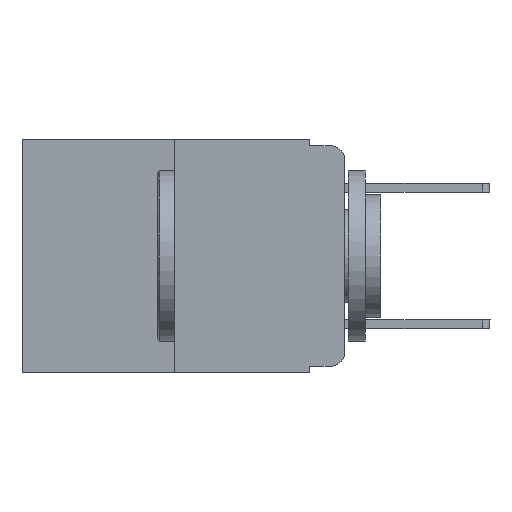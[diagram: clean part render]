
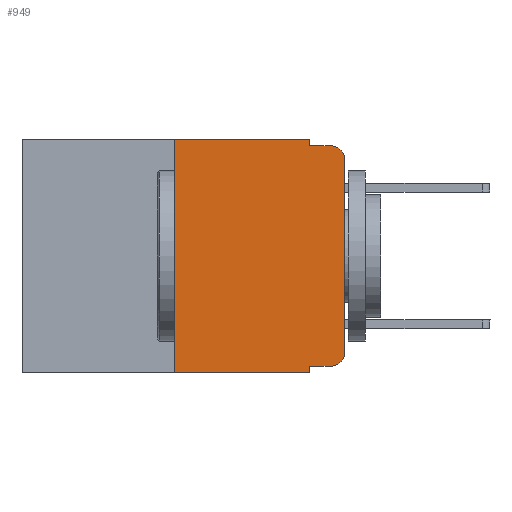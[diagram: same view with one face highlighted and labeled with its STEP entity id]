
A CAD part, left-side view. The second image highlights one B-rep face of the part: STEP entity #949.
In plain terms, the highlighted planar face has unit normal (-1, 0, 0).
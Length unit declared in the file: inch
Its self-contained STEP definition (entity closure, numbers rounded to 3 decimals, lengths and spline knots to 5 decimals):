
#82 = PLANE ( 'NONE',  #6719 ) ;
#690 = CARTESIAN_POINT ( 'NONE',  ( 0., 0.25, 0. ) ) ;
#942 = EDGE_CURVE ( 'NONE', #7728, #4153, #3544, .T. ) ;
#946 = VECTOR ( 'NONE', #10002, 39.37008 ) ;
#949 = ADVANCED_FACE ( 'NONE', ( #10896 ), #82, .F. ) ;
#1170 = VERTEX_POINT ( 'NONE', #7969 ) ;
#1333 = CARTESIAN_POINT ( 'NONE',  ( 0., 0.473, 0. ) ) ;
#1554 = ORIENTED_EDGE ( 'NONE', *, *, #13629, .T. ) ;
#1959 = EDGE_CURVE ( 'NONE', #1170, #15114, #11874, .T. ) ;
#1982 = CARTESIAN_POINT ( 'NONE',  ( 0., 0.02, -0.333 ) ) ;
#2092 = EDGE_CURVE ( 'NONE', #14401, #10902, #7613, .T. ) ;
#2236 = CARTESIAN_POINT ( 'NONE',  ( 0., 0.473, -0.343 ) ) ;
#2256 = ORIENTED_EDGE ( 'NONE', *, *, #4813, .F. ) ;
#2295 = VERTEX_POINT ( 'NONE', #6242 ) ;
#2588 = DIRECTION ( 'NONE',  ( 0., 0., -1. ) ) ;
#2634 = CARTESIAN_POINT ( 'NONE',  ( 0., 0.473, 0. ) ) ;
#2963 = LINE ( 'NONE', #7412, #11364 ) ;
#3075 = VECTOR ( 'NONE', #16510, 39.37008 ) ;
#3254 = CARTESIAN_POINT ( 'NONE',  ( 0., 0.051, -0.01 ) ) ;
#3415 = EDGE_CURVE ( 'NONE', #4444, #14196, #16732, .T. ) ;
#3544 = LINE ( 'NONE', #13118, #12304 ) ;
#3680 = ORIENTED_EDGE ( 'NONE', *, *, #2092, .F. ) ;
#3796 = AXIS2_PLACEMENT_3D ( 'NONE', #14448, #11604, #2588 ) ;
#3921 = EDGE_LOOP ( 'NONE', ( #6752, #1554, #2256, #13914, #3680, #6070, #8173, #13683, #13989, #15368 ) ) ;
#4153 = VERTEX_POINT ( 'NONE', #6490 ) ;
#4444 = VERTEX_POINT ( 'NONE', #15946 ) ;
#4813 = EDGE_CURVE ( 'NONE', #6234, #2295, #2963, .T. ) ;
#5033 = CARTESIAN_POINT ( 'NONE',  ( 0., 0.051, -0.343 ) ) ;
#5127 = CIRCLE ( 'NONE', #14091, 0.02 ) ;
#5692 = VECTOR ( 'NONE', #6187, 39.37008 ) ;
#6070 = ORIENTED_EDGE ( 'NONE', *, *, #13363, .F. ) ;
#6122 = DIRECTION ( 'NONE',  ( -1., 0., 0. ) ) ;
#6187 = DIRECTION ( 'NONE',  ( 0., -1., 0. ) ) ;
#6234 = VERTEX_POINT ( 'NONE', #3254 ) ;
#6242 = CARTESIAN_POINT ( 'NONE',  ( 0., 0.02, -0.01 ) ) ;
#6354 = DIRECTION ( 'NONE',  ( 0., 0., -1. ) ) ;
#6490 = CARTESIAN_POINT ( 'NONE',  ( 0., 0., -0.03 ) ) ;
#6719 = AXIS2_PLACEMENT_3D ( 'NONE', #1333, #11689, #10480 ) ;
#6752 = ORIENTED_EDGE ( 'NONE', *, *, #942, .T. ) ;
#6802 = LINE ( 'NONE', #9765, #16832 ) ;
#7412 = CARTESIAN_POINT ( 'NONE',  ( 0., 0.051, -0.01 ) ) ;
#7445 = CARTESIAN_POINT ( 'NONE',  ( 0., 0.02, -0.313 ) ) ;
#7564 = CARTESIAN_POINT ( 'NONE',  ( 0., 0.051, 0. ) ) ;
#7613 = LINE ( 'NONE', #2634, #3075 ) ;
#7728 = VERTEX_POINT ( 'NONE', #14671 ) ;
#7969 = CARTESIAN_POINT ( 'NONE',  ( 0., 0.051, -0.333 ) ) ;
#8173 = ORIENTED_EDGE ( 'NONE', *, *, #3415, .T. ) ;
#8855 = DIRECTION ( 'NONE',  ( 0., -1., 0. ) ) ;
#9109 = LINE ( 'NONE', #690, #946 ) ;
#9646 = EDGE_CURVE ( 'NONE', #1170, #14196, #6802, .T. ) ;
#9765 = CARTESIAN_POINT ( 'NONE',  ( 0., 0.051, 0. ) ) ;
#10002 = DIRECTION ( 'NONE',  ( 0., 0., 1. ) ) ;
#10020 = CARTESIAN_POINT ( 'NONE',  ( 0., 0.051, 0. ) ) ;
#10300 = EDGE_CURVE ( 'NONE', #10902, #6234, #16820, .T. ) ;
#10480 = DIRECTION ( 'NONE',  ( 0., 0., -1. ) ) ;
#10896 = FACE_OUTER_BOUND ( 'NONE', #3921, .T. ) ;
#10902 = VERTEX_POINT ( 'NONE', #10020 ) ;
#11092 = DIRECTION ( 'NONE',  ( 0., 0., -1. ) ) ;
#11359 = DIRECTION ( 'NONE',  ( 0., 0., -1. ) ) ;
#11364 = VECTOR ( 'NONE', #14184, 39.37008 ) ;
#11604 = DIRECTION ( 'NONE',  ( -1., 0., 0. ) ) ;
#11689 = DIRECTION ( 'NONE',  ( 1., 0., 0. ) ) ;
#11801 = CARTESIAN_POINT ( 'NONE',  ( 0., 0.25, 0. ) ) ;
#11874 = LINE ( 'NONE', #16631, #13109 ) ;
#12152 = CIRCLE ( 'NONE', #3796, 0.02 ) ;
#12153 = EDGE_CURVE ( 'NONE', #15114, #7728, #5127, .T. ) ;
#12304 = VECTOR ( 'NONE', #15807, 39.37008 ) ;
#13109 = VECTOR ( 'NONE', #8855, 39.37008 ) ;
#13118 = CARTESIAN_POINT ( 'NONE',  ( 0., 0., 0. ) ) ;
#13363 = EDGE_CURVE ( 'NONE', #4444, #14401, #9109, .T. ) ;
#13629 = EDGE_CURVE ( 'NONE', #4153, #2295, #12152, .T. ) ;
#13683 = ORIENTED_EDGE ( 'NONE', *, *, #9646, .F. ) ;
#13914 = ORIENTED_EDGE ( 'NONE', *, *, #10300, .F. ) ;
#13989 = ORIENTED_EDGE ( 'NONE', *, *, #1959, .T. ) ;
#14091 = AXIS2_PLACEMENT_3D ( 'NONE', #7445, #6122, #11359 ) ;
#14184 = DIRECTION ( 'NONE',  ( 0., -1., 0. ) ) ;
#14196 = VERTEX_POINT ( 'NONE', #5033 ) ;
#14401 = VERTEX_POINT ( 'NONE', #11801 ) ;
#14448 = CARTESIAN_POINT ( 'NONE',  ( 0., 0.02, -0.03 ) ) ;
#14543 = VECTOR ( 'NONE', #6354, 39.37008 ) ;
#14671 = CARTESIAN_POINT ( 'NONE',  ( 0., 0., -0.313 ) ) ;
#15114 = VERTEX_POINT ( 'NONE', #1982 ) ;
#15368 = ORIENTED_EDGE ( 'NONE', *, *, #12153, .T. ) ;
#15807 = DIRECTION ( 'NONE',  ( 0., 0., 1. ) ) ;
#15946 = CARTESIAN_POINT ( 'NONE',  ( 0., 0.25, -0.343 ) ) ;
#16510 = DIRECTION ( 'NONE',  ( 0., -1., 0. ) ) ;
#16631 = CARTESIAN_POINT ( 'NONE',  ( 0., 0.051, -0.333 ) ) ;
#16732 = LINE ( 'NONE', #2236, #5692 ) ;
#16820 = LINE ( 'NONE', #7564, #14543 ) ;
#16832 = VECTOR ( 'NONE', #11092, 39.37008 ) ;
